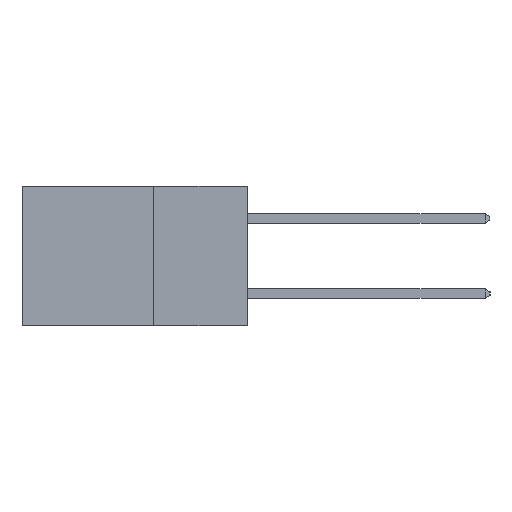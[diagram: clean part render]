
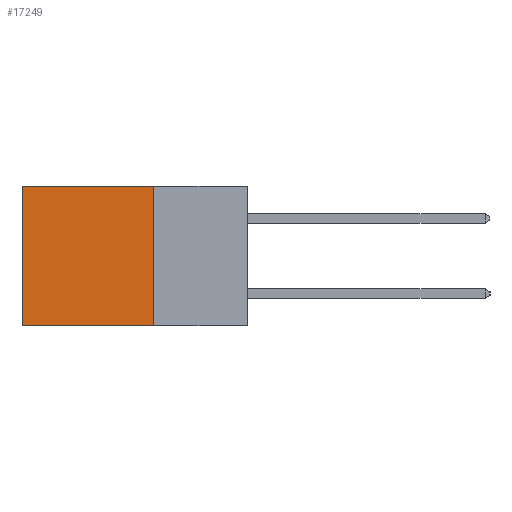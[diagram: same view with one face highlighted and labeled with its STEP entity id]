
A CAD part, left-side view. The second image highlights one B-rep face of the part: STEP entity #17249.
In plain terms, the highlighted planar face has unit normal (-1, 0, 0).
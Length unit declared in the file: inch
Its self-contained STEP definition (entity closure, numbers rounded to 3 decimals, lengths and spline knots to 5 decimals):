
#689 = LINE ( 'NONE', #12498, #16157 ) ;
#3199 = VERTEX_POINT ( 'NONE', #4738 ) ;
#3821 = EDGE_CURVE ( 'NONE', #5226, #8486, #689, .T. ) ;
#4738 = CARTESIAN_POINT ( 'NONE',  ( 0.2615, 0.6, 0. ) ) ;
#5226 = VERTEX_POINT ( 'NONE', #12189 ) ;
#6114 = CARTESIAN_POINT ( 'NONE',  ( 0.2615, 0.25, 0. ) ) ;
#6158 = VECTOR ( 'NONE', #16143, 39.37008 ) ;
#6399 = PLANE ( 'NONE',  #17868 ) ;
#8486 = VERTEX_POINT ( 'NONE', #24369 ) ;
#9337 = FACE_OUTER_BOUND ( 'NONE', #10017, .T. ) ;
#9550 = LINE ( 'NONE', #23704, #24880 ) ;
#9657 = CARTESIAN_POINT ( 'NONE',  ( 0.2615, 0.25, -0.37 ) ) ;
#10017 = EDGE_LOOP ( 'NONE', ( #10561, #25589, #11770, #24214 ) ) ;
#10433 = DIRECTION ( 'NONE',  ( 1., 0., 0. ) ) ;
#10561 = ORIENTED_EDGE ( 'NONE', *, *, #19989, .T. ) ;
#11770 = ORIENTED_EDGE ( 'NONE', *, *, #24508, .F. ) ;
#11877 = LINE ( 'NONE', #9657, #17841 ) ;
#12189 = CARTESIAN_POINT ( 'NONE',  ( 0.2615, 0.25, -0.37 ) ) ;
#12396 = DIRECTION ( 'NONE',  ( 0., 1., 0. ) ) ;
#12498 = CARTESIAN_POINT ( 'NONE',  ( 0.2615, 0.25, -0.37 ) ) ;
#12762 = LINE ( 'NONE', #6114, #6158 ) ;
#13251 = EDGE_CURVE ( 'NONE', #23130, #3199, #12762, .T. ) ;
#16143 = DIRECTION ( 'NONE',  ( 0., 1., 0. ) ) ;
#16157 = VECTOR ( 'NONE', #12396, 39.37008 ) ;
#17249 = ADVANCED_FACE ( 'NONE', ( #9337 ), #6399, .F. ) ;
#17720 = DIRECTION ( 'NONE',  ( 0., 0., -1. ) ) ;
#17841 = VECTOR ( 'NONE', #23680, 39.37008 ) ;
#17868 = AXIS2_PLACEMENT_3D ( 'NONE', #22482, #10433, #24482 ) ;
#19989 = EDGE_CURVE ( 'NONE', #3199, #8486, #9550, .T. ) ;
#21297 = CARTESIAN_POINT ( 'NONE',  ( 0.2615, 0.25, 0. ) ) ;
#22482 = CARTESIAN_POINT ( 'NONE',  ( 0.2615, 0.25, -0.37 ) ) ;
#23130 = VERTEX_POINT ( 'NONE', #21297 ) ;
#23680 = DIRECTION ( 'NONE',  ( 0., 0., -1. ) ) ;
#23704 = CARTESIAN_POINT ( 'NONE',  ( 0.2615, 0.6, -0.37 ) ) ;
#24214 = ORIENTED_EDGE ( 'NONE', *, *, #13251, .T. ) ;
#24369 = CARTESIAN_POINT ( 'NONE',  ( 0.2615, 0.6, -0.37 ) ) ;
#24482 = DIRECTION ( 'NONE',  ( 0., 0., -1. ) ) ;
#24508 = EDGE_CURVE ( 'NONE', #23130, #5226, #11877, .T. ) ;
#24880 = VECTOR ( 'NONE', #17720, 39.37008 ) ;
#25589 = ORIENTED_EDGE ( 'NONE', *, *, #3821, .F. ) ;
